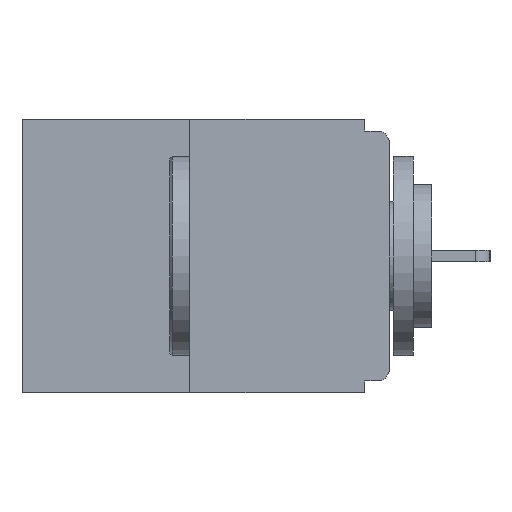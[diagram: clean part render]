
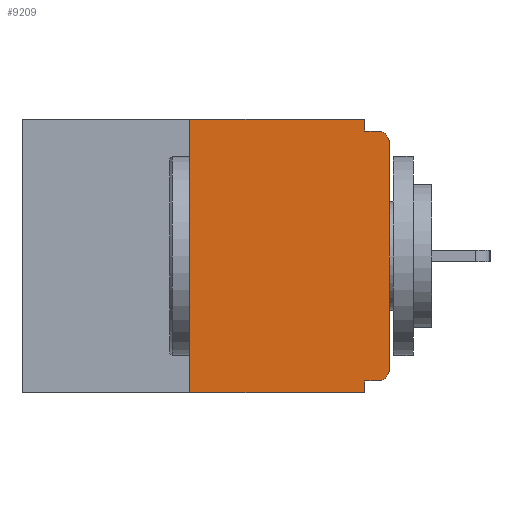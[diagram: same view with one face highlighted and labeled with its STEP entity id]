
A CAD part, left-side view. The second image highlights one B-rep face of the part: STEP entity #9209.
In plain terms, the highlighted planar face has unit normal (-1, 0, 0).
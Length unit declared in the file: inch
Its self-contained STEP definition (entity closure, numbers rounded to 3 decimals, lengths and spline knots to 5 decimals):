
#448 = CARTESIAN_POINT ( 'NONE',  ( 0., 0.25, -0.343 ) ) ;
#583 = EDGE_CURVE ( 'NONE', #16863, #11332, #11423, .T. ) ;
#1035 = LINE ( 'NONE', #6401, #3310 ) ;
#1105 = DIRECTION ( 'NONE',  ( 0., 0., -1. ) ) ;
#1452 = FACE_OUTER_BOUND ( 'NONE', #19834, .T. ) ;
#1596 = VECTOR ( 'NONE', #11400, 39.37008 ) ;
#1638 = CARTESIAN_POINT ( 'NONE',  ( 0., 0., -0.015 ) ) ;
#1668 = VECTOR ( 'NONE', #8159, 39.37008 ) ;
#1854 = DIRECTION ( 'NONE',  ( 0., 0., 1. ) ) ;
#2080 = ORIENTED_EDGE ( 'NONE', *, *, #2162, .T. ) ;
#2162 = EDGE_CURVE ( 'NONE', #19053, #10775, #13322, .T. ) ;
#2787 = AXIS2_PLACEMENT_3D ( 'NONE', #11372, #16993, #11609 ) ;
#3244 = VERTEX_POINT ( 'NONE', #16297 ) ;
#3310 = VECTOR ( 'NONE', #12271, 39.37008 ) ;
#3402 = EDGE_CURVE ( 'NONE', #21372, #10775, #18499, .T. ) ;
#3416 = VERTEX_POINT ( 'NONE', #3965 ) ;
#3965 = CARTESIAN_POINT ( 'NONE',  ( 0., 0.25, 0. ) ) ;
#4088 = VERTEX_POINT ( 'NONE', #13703 ) ;
#4601 = LINE ( 'NONE', #9766, #1668 ) ;
#4755 = EDGE_CURVE ( 'NONE', #3416, #14434, #20703, .T. ) ;
#5124 = CARTESIAN_POINT ( 'NONE',  ( 0., 0., -0.328 ) ) ;
#5561 = EDGE_CURVE ( 'NONE', #16863, #3416, #14818, .T. ) ;
#5672 = DIRECTION ( 'NONE',  ( 0., -1., 0. ) ) ;
#5851 = ORIENTED_EDGE ( 'NONE', *, *, #5899, .T. ) ;
#5899 = EDGE_CURVE ( 'NONE', #4088, #7857, #10285, .T. ) ;
#6140 = LINE ( 'NONE', #15078, #22935 ) ;
#6389 = EDGE_CURVE ( 'NONE', #7857, #19053, #6140, .T. ) ;
#6401 = CARTESIAN_POINT ( 'NONE',  ( 0., 0.031, -0.343 ) ) ;
#6815 = CARTESIAN_POINT ( 'NONE',  ( 0., 0.015, -0.313 ) ) ;
#6974 = VECTOR ( 'NONE', #1854, 39.37008 ) ;
#7822 = VECTOR ( 'NONE', #14433, 39.37008 ) ;
#7857 = VERTEX_POINT ( 'NONE', #23169 ) ;
#8049 = ORIENTED_EDGE ( 'NONE', *, *, #583, .T. ) ;
#8159 = DIRECTION ( 'NONE',  ( 0., 0., -1. ) ) ;
#8161 = CARTESIAN_POINT ( 'NONE',  ( 0., 0., -0.03 ) ) ;
#8299 = EDGE_CURVE ( 'NONE', #4088, #3244, #14799, .T. ) ;
#8647 = CARTESIAN_POINT ( 'NONE',  ( 0., 0.015, -0.015 ) ) ;
#8780 = DIRECTION ( 'NONE',  ( 1., 0., 0. ) ) ;
#9209 = ADVANCED_FACE ( 'NONE', ( #1452 ), #12103, .F. ) ;
#9571 = DIRECTION ( 'NONE',  ( 0., -1., 0. ) ) ;
#9766 = CARTESIAN_POINT ( 'NONE',  ( 0., 0.031, 0. ) ) ;
#10285 = CIRCLE ( 'NONE', #21608, 0.015 ) ;
#10775 = VERTEX_POINT ( 'NONE', #8647 ) ;
#11332 = VERTEX_POINT ( 'NONE', #19736 ) ;
#11372 = CARTESIAN_POINT ( 'NONE',  ( 0., 0.015, -0.03 ) ) ;
#11383 = CARTESIAN_POINT ( 'NONE',  ( 0., 0.25, 0. ) ) ;
#11400 = DIRECTION ( 'NONE',  ( 0., -1., 0. ) ) ;
#11423 = LINE ( 'NONE', #22785, #19483 ) ;
#11609 = DIRECTION ( 'NONE',  ( 0., 0., -1. ) ) ;
#11664 = DIRECTION ( 'NONE',  ( 0., 0., 1. ) ) ;
#12103 = PLANE ( 'NONE',  #15198 ) ;
#12271 = DIRECTION ( 'NONE',  ( 0., 0., -1. ) ) ;
#12621 = CARTESIAN_POINT ( 'NONE',  ( 0., 0.031, 0. ) ) ;
#13322 = CIRCLE ( 'NONE', #2787, 0.015 ) ;
#13703 = CARTESIAN_POINT ( 'NONE',  ( 0., 0.015, -0.328 ) ) ;
#14020 = ORIENTED_EDGE ( 'NONE', *, *, #17633, .F. ) ;
#14245 = ORIENTED_EDGE ( 'NONE', *, *, #8299, .F. ) ;
#14433 = DIRECTION ( 'NONE',  ( 0., 1., 0. ) ) ;
#14434 = VERTEX_POINT ( 'NONE', #12621 ) ;
#14799 = LINE ( 'NONE', #5124, #7822 ) ;
#14818 = LINE ( 'NONE', #11383, #6974 ) ;
#14840 = CARTESIAN_POINT ( 'NONE',  ( 0., 0.46, 0. ) ) ;
#15078 = CARTESIAN_POINT ( 'NONE',  ( 0., 0., 0. ) ) ;
#15198 = AXIS2_PLACEMENT_3D ( 'NONE', #23566, #8780, #1105 ) ;
#15734 = ORIENTED_EDGE ( 'NONE', *, *, #20932, .F. ) ;
#16016 = DIRECTION ( 'NONE',  ( -1., 0., 0. ) ) ;
#16297 = CARTESIAN_POINT ( 'NONE',  ( 0., 0.031, -0.328 ) ) ;
#16726 = ORIENTED_EDGE ( 'NONE', *, *, #6389, .T. ) ;
#16863 = VERTEX_POINT ( 'NONE', #448 ) ;
#16993 = DIRECTION ( 'NONE',  ( -1., 0., 0. ) ) ;
#17633 = EDGE_CURVE ( 'NONE', #14434, #21372, #4601, .T. ) ;
#18499 = LINE ( 'NONE', #1638, #1596 ) ;
#19053 = VERTEX_POINT ( 'NONE', #8161 ) ;
#19143 = VECTOR ( 'NONE', #9571, 39.37008 ) ;
#19483 = VECTOR ( 'NONE', #5672, 39.37008 ) ;
#19736 = CARTESIAN_POINT ( 'NONE',  ( 0., 0.031, -0.343 ) ) ;
#19834 = EDGE_LOOP ( 'NONE', ( #23312, #23142, #8049, #15734, #14245, #5851, #16726, #2080, #21429, #14020 ) ) ;
#20032 = DIRECTION ( 'NONE',  ( 0., 0., -1. ) ) ;
#20703 = LINE ( 'NONE', #14840, #19143 ) ;
#20932 = EDGE_CURVE ( 'NONE', #3244, #11332, #1035, .T. ) ;
#21372 = VERTEX_POINT ( 'NONE', #21649 ) ;
#21429 = ORIENTED_EDGE ( 'NONE', *, *, #3402, .F. ) ;
#21608 = AXIS2_PLACEMENT_3D ( 'NONE', #6815, #16016, #20032 ) ;
#21649 = CARTESIAN_POINT ( 'NONE',  ( 0., 0.031, -0.015 ) ) ;
#22785 = CARTESIAN_POINT ( 'NONE',  ( 0., 0.46, -0.343 ) ) ;
#22935 = VECTOR ( 'NONE', #11664, 39.37008 ) ;
#23142 = ORIENTED_EDGE ( 'NONE', *, *, #5561, .F. ) ;
#23169 = CARTESIAN_POINT ( 'NONE',  ( 0., 0., -0.313 ) ) ;
#23312 = ORIENTED_EDGE ( 'NONE', *, *, #4755, .F. ) ;
#23566 = CARTESIAN_POINT ( 'NONE',  ( 0., 0.46, 0. ) ) ;
